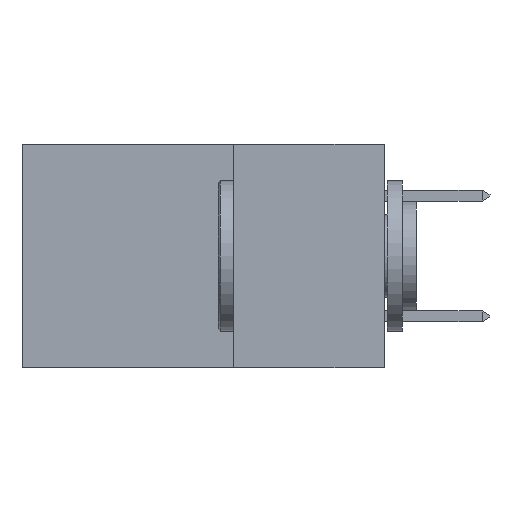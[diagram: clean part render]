
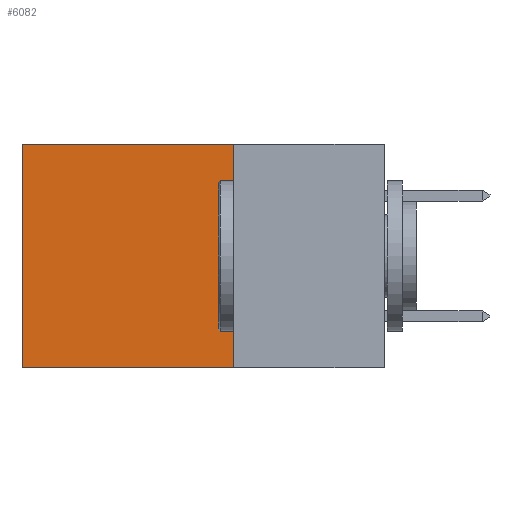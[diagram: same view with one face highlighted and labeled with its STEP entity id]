
A CAD part, left-side view. The second image highlights one B-rep face of the part: STEP entity #6082.
In plain terms, the highlighted planar face has unit normal (-1, 0, 0).
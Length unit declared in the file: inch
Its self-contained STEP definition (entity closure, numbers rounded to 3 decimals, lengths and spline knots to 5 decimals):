
#101 = VECTOR ( 'NONE', #12617, 39.37008 ) ;
#145 = CARTESIAN_POINT ( 'NONE',  ( 0.2875, 0.6, 0. ) ) ;
#2059 = EDGE_CURVE ( 'NONE', #6796, #6471, #8065, .T. ) ;
#2395 = LINE ( 'NONE', #2473, #10472 ) ;
#2473 = CARTESIAN_POINT ( 'NONE',  ( 0.2875, 0.25, 0. ) ) ;
#2900 = CARTESIAN_POINT ( 'NONE',  ( 0.2875, 0.25, 0. ) ) ;
#3607 = VERTEX_POINT ( 'NONE', #145 ) ;
#3927 = CARTESIAN_POINT ( 'NONE',  ( 0.2875, 0.6, -0.37 ) ) ;
#4688 = DIRECTION ( 'NONE',  ( 0., 0., -1. ) ) ;
#4764 = ORIENTED_EDGE ( 'NONE', *, *, #11503, .T. ) ;
#5084 = ORIENTED_EDGE ( 'NONE', *, *, #2059, .F. ) ;
#5241 = VERTEX_POINT ( 'NONE', #2900 ) ;
#5426 = CARTESIAN_POINT ( 'NONE',  ( 0.2875, 0.25, 0. ) ) ;
#5887 = AXIS2_PLACEMENT_3D ( 'NONE', #5426, #13552, #7516 ) ;
#6082 = ADVANCED_FACE ( 'NONE', ( #9444 ), #12623, .F. ) ;
#6240 = EDGE_CURVE ( 'NONE', #5241, #6796, #7161, .T. ) ;
#6471 = VERTEX_POINT ( 'NONE', #3927 ) ;
#6529 = VECTOR ( 'NONE', #12339, 39.37008 ) ;
#6796 = VERTEX_POINT ( 'NONE', #8604 ) ;
#7161 = LINE ( 'NONE', #11912, #7473 ) ;
#7473 = VECTOR ( 'NONE', #4688, 39.37008 ) ;
#7516 = DIRECTION ( 'NONE',  ( 0., 0., -1. ) ) ;
#8065 = LINE ( 'NONE', #12664, #101 ) ;
#8250 = CARTESIAN_POINT ( 'NONE',  ( 0.2875, 0.6, 0. ) ) ;
#8518 = EDGE_CURVE ( 'NONE', #5241, #3607, #2395, .T. ) ;
#8604 = CARTESIAN_POINT ( 'NONE',  ( 0.2875, 0.25, -0.37 ) ) ;
#9444 = FACE_OUTER_BOUND ( 'NONE', #9550, .T. ) ;
#9550 = EDGE_LOOP ( 'NONE', ( #4764, #5084, #13238, #13526 ) ) ;
#10472 = VECTOR ( 'NONE', #10895, 39.37008 ) ;
#10895 = DIRECTION ( 'NONE',  ( 0., 1., 0. ) ) ;
#11503 = EDGE_CURVE ( 'NONE', #3607, #6471, #11985, .T. ) ;
#11912 = CARTESIAN_POINT ( 'NONE',  ( 0.2875, 0.25, 0. ) ) ;
#11985 = LINE ( 'NONE', #8250, #6529 ) ;
#12339 = DIRECTION ( 'NONE',  ( 0., 0., -1. ) ) ;
#12617 = DIRECTION ( 'NONE',  ( 0., 1., 0. ) ) ;
#12623 = PLANE ( 'NONE',  #5887 ) ;
#12664 = CARTESIAN_POINT ( 'NONE',  ( 0.2875, 0.25, -0.37 ) ) ;
#13238 = ORIENTED_EDGE ( 'NONE', *, *, #6240, .F. ) ;
#13526 = ORIENTED_EDGE ( 'NONE', *, *, #8518, .T. ) ;
#13552 = DIRECTION ( 'NONE',  ( 1., 0., 0. ) ) ;
